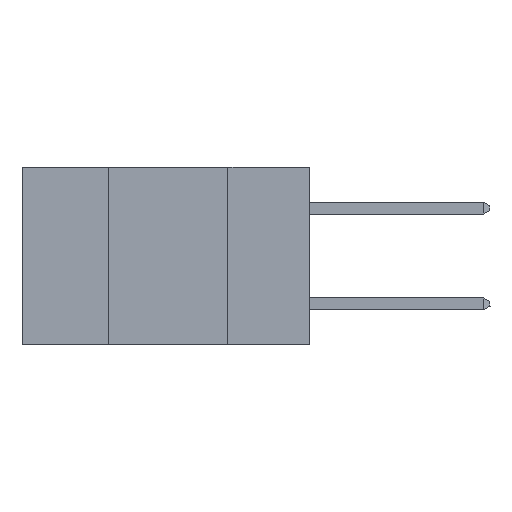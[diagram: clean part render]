
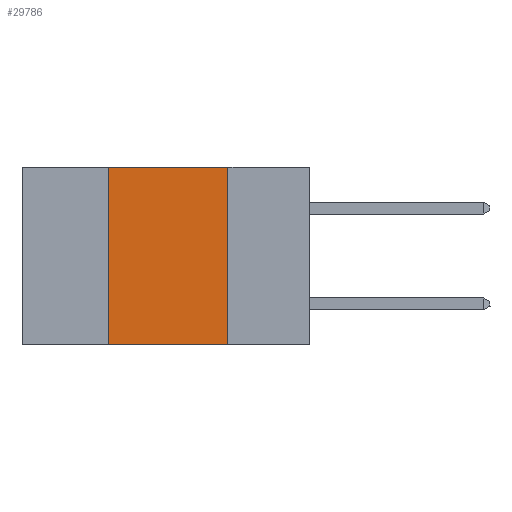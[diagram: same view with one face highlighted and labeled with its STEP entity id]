
A CAD part, left-side view. The second image highlights one B-rep face of the part: STEP entity #29786.
In plain terms, the highlighted planar face has unit normal (-1, 0, 0).
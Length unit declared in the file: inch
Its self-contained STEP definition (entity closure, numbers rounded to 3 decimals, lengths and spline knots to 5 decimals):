
#118 = EDGE_CURVE ( 'NONE', #19679, #17284, #8697, .T. ) ;
#391 = EDGE_CURVE ( 'NONE', #19679, #31583, #7563, .T. ) ;
#2393 = LINE ( 'NONE', #30941, #10319 ) ;
#2746 = EDGE_CURVE ( 'NONE', #9369, #17284, #2393, .T. ) ;
#4478 = PLANE ( 'NONE',  #16608 ) ;
#4640 = CARTESIAN_POINT ( 'NONE',  ( 0., 0.42, 0. ) ) ;
#4987 = DIRECTION ( 'NONE',  ( 0., 0., 1. ) ) ;
#4997 = CARTESIAN_POINT ( 'NONE',  ( 0., 0.6, 0. ) ) ;
#5581 = CARTESIAN_POINT ( 'NONE',  ( 0., 0.6, -0.37 ) ) ;
#7192 = VECTOR ( 'NONE', #4987, 39.37008 ) ;
#7281 = ORIENTED_EDGE ( 'NONE', *, *, #118, .T. ) ;
#7563 = LINE ( 'NONE', #4640, #7192 ) ;
#8076 = DIRECTION ( 'NONE',  ( 0., 0., -1. ) ) ;
#8697 = LINE ( 'NONE', #5581, #16570 ) ;
#9369 = VERTEX_POINT ( 'NONE', #13293 ) ;
#10319 = VECTOR ( 'NONE', #8076, 39.37008 ) ;
#10330 = CARTESIAN_POINT ( 'NONE',  ( 0., 0.17, -0.37 ) ) ;
#10506 = DIRECTION ( 'NONE',  ( 1., 0., 0. ) ) ;
#13293 = CARTESIAN_POINT ( 'NONE',  ( 0., 0.17, 0. ) ) ;
#16570 = VECTOR ( 'NONE', #33380, 39.37008 ) ;
#16608 = AXIS2_PLACEMENT_3D ( 'NONE', #4997, #10506, #29718 ) ;
#17284 = VERTEX_POINT ( 'NONE', #10330 ) ;
#19679 = VERTEX_POINT ( 'NONE', #32553 ) ;
#20476 = ORIENTED_EDGE ( 'NONE', *, *, #391, .F. ) ;
#20845 = ORIENTED_EDGE ( 'NONE', *, *, #28362, .F. ) ;
#22655 = EDGE_LOOP ( 'NONE', ( #26264, #20845, #20476, #7281 ) ) ;
#23683 = CARTESIAN_POINT ( 'NONE',  ( 0., 0.6, 0. ) ) ;
#26230 = DIRECTION ( 'NONE',  ( 0., -1., 0. ) ) ;
#26264 = ORIENTED_EDGE ( 'NONE', *, *, #2746, .F. ) ;
#28362 = EDGE_CURVE ( 'NONE', #31583, #9369, #32069, .T. ) ;
#29718 = DIRECTION ( 'NONE',  ( 0., 0., -1. ) ) ;
#29786 = ADVANCED_FACE ( 'NONE', ( #32462 ), #4478, .F. ) ;
#30054 = CARTESIAN_POINT ( 'NONE',  ( 0., 0.42, 0. ) ) ;
#30941 = CARTESIAN_POINT ( 'NONE',  ( 0., 0.17, 0. ) ) ;
#31583 = VERTEX_POINT ( 'NONE', #30054 ) ;
#32069 = LINE ( 'NONE', #23683, #33992 ) ;
#32462 = FACE_OUTER_BOUND ( 'NONE', #22655, .T. ) ;
#32553 = CARTESIAN_POINT ( 'NONE',  ( 0., 0.42, -0.37 ) ) ;
#33380 = DIRECTION ( 'NONE',  ( 0., -1., 0. ) ) ;
#33992 = VECTOR ( 'NONE', #26230, 39.37008 ) ;
